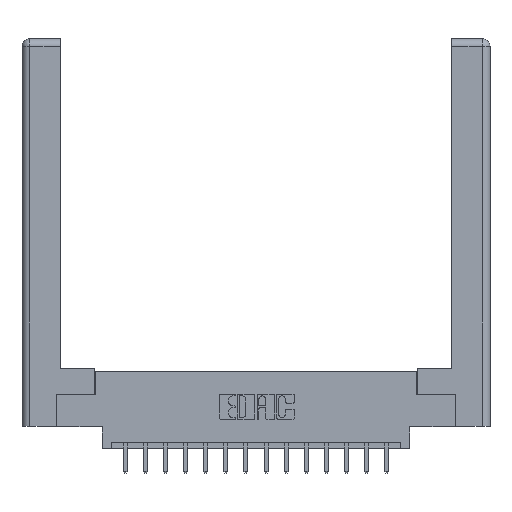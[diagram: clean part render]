
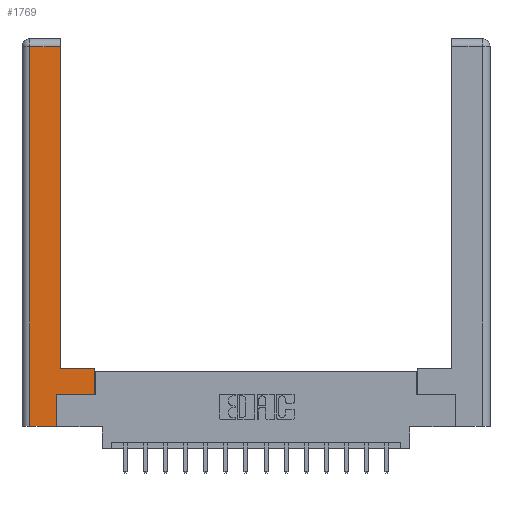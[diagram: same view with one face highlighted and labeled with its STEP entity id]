
A CAD part, top view. The second image highlights one B-rep face of the part: STEP entity #1769.
In plain terms, the highlighted planar face has unit normal (0, 0, 1).
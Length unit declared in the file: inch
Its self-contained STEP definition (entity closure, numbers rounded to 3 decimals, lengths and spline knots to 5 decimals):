
#436 = CARTESIAN_POINT ( 'NONE',  ( 0.295, 0.45, 0. ) ) ;
#1278 = CARTESIAN_POINT ( 'NONE',  ( 0.0615, 2.94, 0. ) ) ;
#1769 = ADVANCED_FACE ( 'NONE', ( #3878 ), #12321, .F. ) ;
#1809 = CARTESIAN_POINT ( 'NONE',  ( 0.295, 2.94, 0. ) ) ;
#1872 = LINE ( 'NONE', #6422, #16156 ) ;
#2258 = ORIENTED_EDGE ( 'NONE', *, *, #4574, .T. ) ;
#2673 = EDGE_CURVE ( 'NONE', #7724, #15096, #13729, .T. ) ;
#3304 = CARTESIAN_POINT ( 'NONE',  ( 0.565, 0.245, 0. ) ) ;
#3341 = LINE ( 'NONE', #15744, #15118 ) ;
#3777 = LINE ( 'NONE', #10205, #12399 ) ;
#3878 = FACE_OUTER_BOUND ( 'NONE', #15767, .T. ) ;
#4415 = CARTESIAN_POINT ( 'NONE',  ( 0.265, 0., 0. ) ) ;
#4431 = CARTESIAN_POINT ( 'NONE',  ( 0., 0., 0. ) ) ;
#4574 = EDGE_CURVE ( 'NONE', #15096, #16524, #10108, .T. ) ;
#4691 = VECTOR ( 'NONE', #7462, 39.37008 ) ;
#4749 = DIRECTION ( 'NONE',  ( 0., 1., 0. ) ) ;
#5160 = CARTESIAN_POINT ( 'NONE',  ( 0.565, 0.45, 0. ) ) ;
#5262 = ORIENTED_EDGE ( 'NONE', *, *, #16338, .T. ) ;
#5648 = CARTESIAN_POINT ( 'NONE',  ( 0.265, 0.245, 0. ) ) ;
#5772 = DIRECTION ( 'NONE',  ( 1., 0., 0. ) ) ;
#5829 = VERTEX_POINT ( 'NONE', #15245 ) ;
#6079 = CARTESIAN_POINT ( 'NONE',  ( 0.565, 0.245, 0. ) ) ;
#6422 = CARTESIAN_POINT ( 'NONE',  ( 0.0615, 2.94, 0. ) ) ;
#6532 = VECTOR ( 'NONE', #11020, 39.37008 ) ;
#6596 = VECTOR ( 'NONE', #5772, 39.37008 ) ;
#6913 = EDGE_CURVE ( 'NONE', #16524, #9902, #16863, .T. ) ;
#7455 = DIRECTION ( 'NONE',  ( 0., -1., 0. ) ) ;
#7462 = DIRECTION ( 'NONE',  ( 1., 0., 0. ) ) ;
#7724 = VERTEX_POINT ( 'NONE', #16627 ) ;
#7788 = ORIENTED_EDGE ( 'NONE', *, *, #6913, .T. ) ;
#7995 = VECTOR ( 'NONE', #7455, 39.37008 ) ;
#8586 = EDGE_CURVE ( 'NONE', #12785, #5829, #10297, .T. ) ;
#8638 = VECTOR ( 'NONE', #15238, 39.37008 ) ;
#8662 = EDGE_CURVE ( 'NONE', #13108, #7724, #9468, .T. ) ;
#8859 = DIRECTION ( 'NONE',  ( 0., 1., 0. ) ) ;
#9468 = LINE ( 'NONE', #12898, #7995 ) ;
#9902 = VERTEX_POINT ( 'NONE', #3304 ) ;
#10108 = LINE ( 'NONE', #16446, #6532 ) ;
#10205 = CARTESIAN_POINT ( 'NONE',  ( 0.565, 0.45, 0. ) ) ;
#10297 = LINE ( 'NONE', #436, #8638 ) ;
#10800 = ORIENTED_EDGE ( 'NONE', *, *, #8662, .T. ) ;
#11020 = DIRECTION ( 'NONE',  ( 0., 1., 0. ) ) ;
#11770 = DIRECTION ( 'NONE',  ( -1., 0., 0. ) ) ;
#11851 = ORIENTED_EDGE ( 'NONE', *, *, #2673, .T. ) ;
#12321 = PLANE ( 'NONE',  #12834 ) ;
#12399 = VECTOR ( 'NONE', #4749, 39.37008 ) ;
#12683 = VERTEX_POINT ( 'NONE', #1809 ) ;
#12785 = VERTEX_POINT ( 'NONE', #5160 ) ;
#12834 = AXIS2_PLACEMENT_3D ( 'NONE', #4431, #13766, #16822 ) ;
#12898 = CARTESIAN_POINT ( 'NONE',  ( 0.0615, 0., 0. ) ) ;
#13108 = VERTEX_POINT ( 'NONE', #1278 ) ;
#13317 = ORIENTED_EDGE ( 'NONE', *, *, #14331, .T. ) ;
#13729 = LINE ( 'NONE', #4415, #6596 ) ;
#13766 = DIRECTION ( 'NONE',  ( 0., 0., -1. ) ) ;
#14331 = EDGE_CURVE ( 'NONE', #9902, #12785, #3777, .T. ) ;
#14640 = ORIENTED_EDGE ( 'NONE', *, *, #8586, .T. ) ;
#15096 = VERTEX_POINT ( 'NONE', #15770 ) ;
#15118 = VECTOR ( 'NONE', #8859, 39.37008 ) ;
#15238 = DIRECTION ( 'NONE',  ( -1., 0., 0. ) ) ;
#15245 = CARTESIAN_POINT ( 'NONE',  ( 0.295, 0.45, 0. ) ) ;
#15744 = CARTESIAN_POINT ( 'NONE',  ( 0.295, 3., 0. ) ) ;
#15767 = EDGE_LOOP ( 'NONE', ( #5262, #16286, #10800, #11851, #2258, #7788, #13317, #14640 ) ) ;
#15770 = CARTESIAN_POINT ( 'NONE',  ( 0.265, 0., 0. ) ) ;
#16156 = VECTOR ( 'NONE', #11770, 39.37008 ) ;
#16286 = ORIENTED_EDGE ( 'NONE', *, *, #16675, .T. ) ;
#16338 = EDGE_CURVE ( 'NONE', #5829, #12683, #3341, .T. ) ;
#16446 = CARTESIAN_POINT ( 'NONE',  ( 0.265, 0.245, 0. ) ) ;
#16524 = VERTEX_POINT ( 'NONE', #5648 ) ;
#16627 = CARTESIAN_POINT ( 'NONE',  ( 0.0615, 0., 0. ) ) ;
#16675 = EDGE_CURVE ( 'NONE', #12683, #13108, #1872, .T. ) ;
#16822 = DIRECTION ( 'NONE',  ( -1., 0., 0. ) ) ;
#16863 = LINE ( 'NONE', #6079, #4691 ) ;
